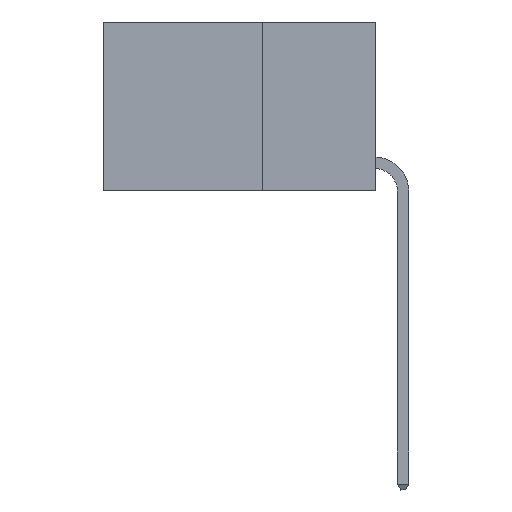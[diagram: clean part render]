
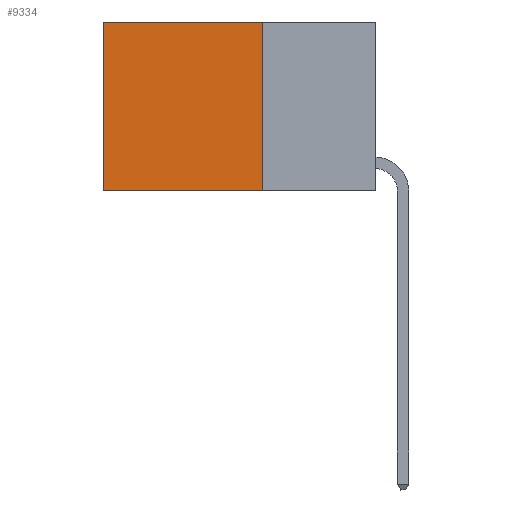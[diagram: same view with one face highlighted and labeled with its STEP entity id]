
A CAD part, left-side view. The second image highlights one B-rep face of the part: STEP entity #9334.
In plain terms, the highlighted planar face has unit normal (-1, 0, 0).
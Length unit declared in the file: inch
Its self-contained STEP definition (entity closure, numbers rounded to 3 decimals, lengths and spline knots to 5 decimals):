
#87 = VECTOR ( 'NONE', #1369, 39.37008 ) ;
#453 = DIRECTION ( 'NONE',  ( 0., 1., 0. ) ) ;
#524 = CARTESIAN_POINT ( 'NONE',  ( 0.2625, 0.6, -0.37 ) ) ;
#1369 = DIRECTION ( 'NONE',  ( 0., 0., -1. ) ) ;
#2061 = LINE ( 'NONE', #4536, #9055 ) ;
#2125 = CARTESIAN_POINT ( 'NONE',  ( 0.2625, 0.25, -0.37 ) ) ;
#2530 = PLANE ( 'NONE',  #5641 ) ;
#3192 = VERTEX_POINT ( 'NONE', #5586 ) ;
#3461 = ORIENTED_EDGE ( 'NONE', *, *, #14780, .F. ) ;
#3830 = EDGE_LOOP ( 'NONE', ( #8192, #9789, #3461, #15797 ) ) ;
#4536 = CARTESIAN_POINT ( 'NONE',  ( 0.2625, 0.25, -0.37 ) ) ;
#4593 = VECTOR ( 'NONE', #453, 39.37008 ) ;
#5527 = CARTESIAN_POINT ( 'NONE',  ( 0.2625, 0.25, 0. ) ) ;
#5586 = CARTESIAN_POINT ( 'NONE',  ( 0.2625, 0.25, 0. ) ) ;
#5641 = AXIS2_PLACEMENT_3D ( 'NONE', #9605, #13370, #7439 ) ;
#6644 = LINE ( 'NONE', #10414, #10234 ) ;
#6728 = LINE ( 'NONE', #5527, #4593 ) ;
#6765 = EDGE_CURVE ( 'NONE', #12912, #13562, #6644, .T. ) ;
#6814 = EDGE_CURVE ( 'NONE', #3192, #12912, #6728, .T. ) ;
#7439 = DIRECTION ( 'NONE',  ( 0., 0., -1. ) ) ;
#7864 = DIRECTION ( 'NONE',  ( 0., 1., 0. ) ) ;
#8192 = ORIENTED_EDGE ( 'NONE', *, *, #6765, .T. ) ;
#8518 = CARTESIAN_POINT ( 'NONE',  ( 0.2625, 0.6, 0. ) ) ;
#9055 = VECTOR ( 'NONE', #7864, 39.37008 ) ;
#9334 = ADVANCED_FACE ( 'NONE', ( #13523 ), #2530, .F. ) ;
#9605 = CARTESIAN_POINT ( 'NONE',  ( 0.2625, 0.25, 0. ) ) ;
#9789 = ORIENTED_EDGE ( 'NONE', *, *, #12482, .F. ) ;
#10234 = VECTOR ( 'NONE', #12914, 39.37008 ) ;
#10414 = CARTESIAN_POINT ( 'NONE',  ( 0.2625, 0.6, 0. ) ) ;
#12371 = LINE ( 'NONE', #15081, #87 ) ;
#12482 = EDGE_CURVE ( 'NONE', #15259, #13562, #2061, .T. ) ;
#12912 = VERTEX_POINT ( 'NONE', #8518 ) ;
#12914 = DIRECTION ( 'NONE',  ( 0., 0., -1. ) ) ;
#13370 = DIRECTION ( 'NONE',  ( 1., 0., 0. ) ) ;
#13523 = FACE_OUTER_BOUND ( 'NONE', #3830, .T. ) ;
#13562 = VERTEX_POINT ( 'NONE', #524 ) ;
#14780 = EDGE_CURVE ( 'NONE', #3192, #15259, #12371, .T. ) ;
#15081 = CARTESIAN_POINT ( 'NONE',  ( 0.2625, 0.25, 0. ) ) ;
#15259 = VERTEX_POINT ( 'NONE', #2125 ) ;
#15797 = ORIENTED_EDGE ( 'NONE', *, *, #6814, .T. ) ;
